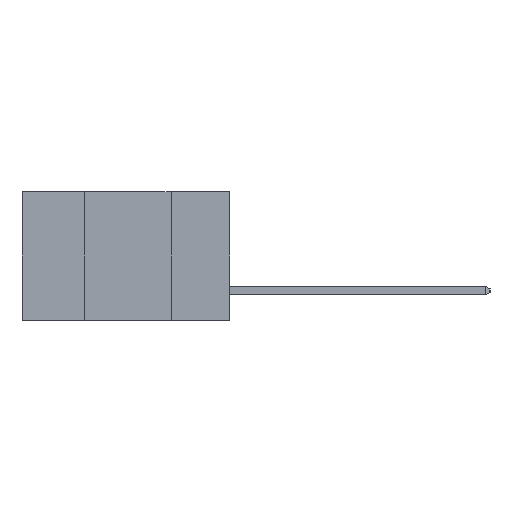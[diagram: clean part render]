
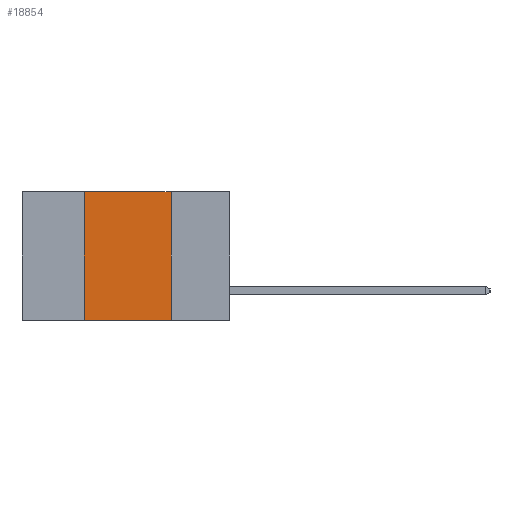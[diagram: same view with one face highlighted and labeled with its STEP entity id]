
A CAD part, left-side view. The second image highlights one B-rep face of the part: STEP entity #18854.
In plain terms, the highlighted planar face has unit normal (-1, 0, 0).
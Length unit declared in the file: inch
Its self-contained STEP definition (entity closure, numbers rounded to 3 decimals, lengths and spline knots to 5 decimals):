
#133 = LINE ( 'NONE', #20519, #20091 ) ;
#1652 = ORIENTED_EDGE ( 'NONE', *, *, #6661, .F. ) ;
#3431 = CARTESIAN_POINT ( 'NONE',  ( 0., 0.17, 0. ) ) ;
#3450 = FACE_OUTER_BOUND ( 'NONE', #23646, .T. ) ;
#4961 = DIRECTION ( 'NONE',  ( 0., -1., 0. ) ) ;
#6661 = EDGE_CURVE ( 'NONE', #11215, #16364, #133, .T. ) ;
#7485 = CARTESIAN_POINT ( 'NONE',  ( 0., 0.6, -0.37 ) ) ;
#7592 = VECTOR ( 'NONE', #30434, 39.37008 ) ;
#8663 = CARTESIAN_POINT ( 'NONE',  ( 0., 0.6, 0. ) ) ;
#9684 = LINE ( 'NONE', #20919, #22556 ) ;
#9733 = AXIS2_PLACEMENT_3D ( 'NONE', #8663, #26530, #11317 ) ;
#11215 = VERTEX_POINT ( 'NONE', #26831 ) ;
#11317 = DIRECTION ( 'NONE',  ( 0., 0., -1. ) ) ;
#12021 = VERTEX_POINT ( 'NONE', #19974 ) ;
#14329 = VERTEX_POINT ( 'NONE', #29665 ) ;
#14606 = LINE ( 'NONE', #7485, #7592 ) ;
#15474 = LINE ( 'NONE', #23321, #28039 ) ;
#15639 = ORIENTED_EDGE ( 'NONE', *, *, #17458, .F. ) ;
#15756 = EDGE_CURVE ( 'NONE', #14329, #12021, #14606, .T. ) ;
#16364 = VERTEX_POINT ( 'NONE', #3431 ) ;
#17229 = ORIENTED_EDGE ( 'NONE', *, *, #15756, .T. ) ;
#17458 = EDGE_CURVE ( 'NONE', #14329, #11215, #15474, .T. ) ;
#18854 = ADVANCED_FACE ( 'NONE', ( #3450 ), #24030, .F. ) ;
#19974 = CARTESIAN_POINT ( 'NONE',  ( 0., 0.17, -0.37 ) ) ;
#20091 = VECTOR ( 'NONE', #4961, 39.37008 ) ;
#20519 = CARTESIAN_POINT ( 'NONE',  ( 0., 0.6, 0. ) ) ;
#20762 = ORIENTED_EDGE ( 'NONE', *, *, #30863, .F. ) ;
#20919 = CARTESIAN_POINT ( 'NONE',  ( 0., 0.17, 0. ) ) ;
#22556 = VECTOR ( 'NONE', #23419, 39.37008 ) ;
#23321 = CARTESIAN_POINT ( 'NONE',  ( 0., 0.42, 0. ) ) ;
#23419 = DIRECTION ( 'NONE',  ( 0., 0., -1. ) ) ;
#23646 = EDGE_LOOP ( 'NONE', ( #20762, #1652, #15639, #17229 ) ) ;
#24030 = PLANE ( 'NONE',  #9733 ) ;
#26530 = DIRECTION ( 'NONE',  ( 1., 0., 0. ) ) ;
#26831 = CARTESIAN_POINT ( 'NONE',  ( 0., 0.42, 0. ) ) ;
#28039 = VECTOR ( 'NONE', #28362, 39.37008 ) ;
#28362 = DIRECTION ( 'NONE',  ( 0., 0., 1. ) ) ;
#29665 = CARTESIAN_POINT ( 'NONE',  ( 0., 0.42, -0.37 ) ) ;
#30434 = DIRECTION ( 'NONE',  ( 0., -1., 0. ) ) ;
#30863 = EDGE_CURVE ( 'NONE', #16364, #12021, #9684, .T. ) ;
